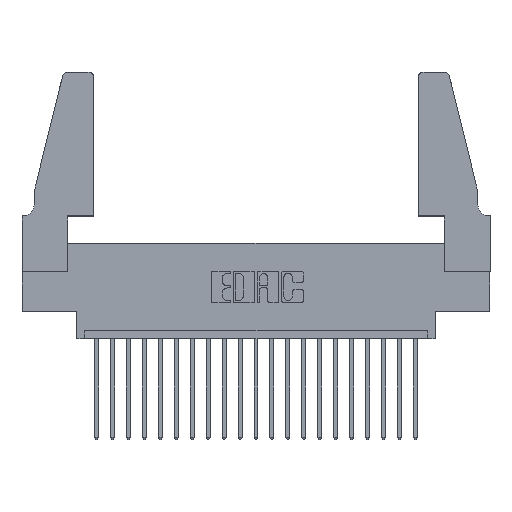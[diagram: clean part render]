
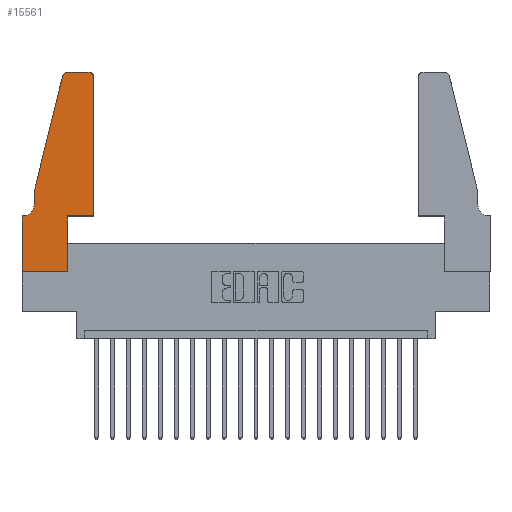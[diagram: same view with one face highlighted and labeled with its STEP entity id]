
A CAD part, top view. The second image highlights one B-rep face of the part: STEP entity #15561.
In plain terms, the highlighted planar face has unit normal (0, 0, 1).
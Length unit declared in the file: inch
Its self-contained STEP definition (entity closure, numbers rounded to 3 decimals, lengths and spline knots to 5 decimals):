
#14 = FACE_OUTER_BOUND ( 'NONE', #16671, .T. ) ;
#288 = CARTESIAN_POINT ( 'NONE',  ( 0., 0., 0.37 ) ) ;
#411 = VERTEX_POINT ( 'NONE', #14215 ) ;
#763 = EDGE_CURVE ( 'NONE', #1324, #10834, #10234, .T. ) ;
#922 = VECTOR ( 'NONE', #19363, 39.37008 ) ;
#1069 = VECTOR ( 'NONE', #16514, 39.37008 ) ;
#1324 = VERTEX_POINT ( 'NONE', #14878 ) ;
#1647 = DIRECTION ( 'NONE',  ( 0., -1., 0. ) ) ;
#1745 = DIRECTION ( 'NONE',  ( 0., 0., 1. ) ) ;
#1915 = DIRECTION ( 'NONE',  ( 1., 0., 0. ) ) ;
#1944 = ORIENTED_EDGE ( 'NONE', *, *, #763, .T. ) ;
#2121 = DIRECTION ( 'NONE',  ( 0., 0., -1. ) ) ;
#2339 = EDGE_CURVE ( 'NONE', #411, #6977, #4981, .T. ) ;
#2357 = CARTESIAN_POINT ( 'NONE',  ( 0.0755, 0.35, 0.37 ) ) ;
#2499 = ORIENTED_EDGE ( 'NONE', *, *, #9506, .T. ) ;
#2658 = ORIENTED_EDGE ( 'NONE', *, *, #4886, .T. ) ;
#2689 = CARTESIAN_POINT ( 'NONE',  ( 0.4205, 1.22, 0.37 ) ) ;
#3113 = VECTOR ( 'NONE', #1647, 39.37008 ) ;
#3152 = CIRCLE ( 'NONE', #9971, 0.03 ) ;
#3331 = DIRECTION ( 'NONE',  ( -1., 0., 0. ) ) ;
#3365 = CIRCLE ( 'NONE', #14687, 0.03 ) ;
#3493 = DIRECTION ( 'NONE',  ( 0., -1., 0. ) ) ;
#3897 = ORIENTED_EDGE ( 'NONE', *, *, #10611, .T. ) ;
#3957 = LINE ( 'NONE', #11464, #922 ) ;
#4036 = LINE ( 'NONE', #2357, #15236 ) ;
#4206 = VERTEX_POINT ( 'NONE', #18642 ) ;
#4477 = ORIENTED_EDGE ( 'NONE', *, *, #12976, .T. ) ;
#4507 = VERTEX_POINT ( 'NONE', #16225 ) ;
#4637 = EDGE_CURVE ( 'NONE', #10834, #4507, #16852, .T. ) ;
#4656 = DIRECTION ( 'NONE',  ( -1., 0., 0. ) ) ;
#4687 = ORIENTED_EDGE ( 'NONE', *, *, #18938, .T. ) ;
#4770 = CARTESIAN_POINT ( 'NONE',  ( 0., 0.35, 0.37 ) ) ;
#4886 = EDGE_CURVE ( 'NONE', #4206, #8396, #3365, .T. ) ;
#4981 = CIRCLE ( 'NONE', #7730, 0.07 ) ;
#5059 = CARTESIAN_POINT ( 'NONE',  ( 0.2865, 0., 0.37 ) ) ;
#5450 = VECTOR ( 'NONE', #19411, 39.37008 ) ;
#5942 = DIRECTION ( 'NONE',  ( 1., 0., 0. ) ) ;
#6318 = CARTESIAN_POINT ( 'NONE',  ( 0.284, 1.22, 0.37 ) ) ;
#6437 = PLANE ( 'NONE',  #16159 ) ;
#6472 = LINE ( 'NONE', #11376, #5450 ) ;
#6556 = DIRECTION ( 'NONE',  ( 0., 1., 0. ) ) ;
#6845 = CARTESIAN_POINT ( 'NONE',  ( 0.0755, 0.5, 0.37 ) ) ;
#6977 = VERTEX_POINT ( 'NONE', #12449 ) ;
#7044 = CARTESIAN_POINT ( 'NONE',  ( 0., 0.35, 0.37 ) ) ;
#7730 = AXIS2_PLACEMENT_3D ( 'NONE', #11514, #2121, #4656 ) ;
#7731 = VECTOR ( 'NONE', #6556, 39.37008 ) ;
#8396 = VERTEX_POINT ( 'NONE', #16308 ) ;
#8478 = LINE ( 'NONE', #6845, #3113 ) ;
#9409 = ORIENTED_EDGE ( 'NONE', *, *, #4637, .T. ) ;
#9506 = EDGE_CURVE ( 'NONE', #6977, #15412, #4036, .T. ) ;
#9590 = LINE ( 'NONE', #17860, #13404 ) ;
#9971 = AXIS2_PLACEMENT_3D ( 'NONE', #2689, #15674, #5942 ) ;
#10210 = DIRECTION ( 'NONE',  ( 1., 0., 0. ) ) ;
#10234 = LINE ( 'NONE', #14750, #1069 ) ;
#10611 = EDGE_CURVE ( 'NONE', #15412, #11707, #9590, .T. ) ;
#10834 = VERTEX_POINT ( 'NONE', #11887 ) ;
#11376 = CARTESIAN_POINT ( 'NONE',  ( 0.0755, 0.5, 0.37 ) ) ;
#11464 = CARTESIAN_POINT ( 'NONE',  ( 0.2865, 0.35, 0.37 ) ) ;
#11514 = CARTESIAN_POINT ( 'NONE',  ( 0.0055, 0.42, 0.37 ) ) ;
#11580 = ORIENTED_EDGE ( 'NONE', *, *, #17772, .T. ) ;
#11686 = ORIENTED_EDGE ( 'NONE', *, *, #12590, .T. ) ;
#11707 = VERTEX_POINT ( 'NONE', #20818 ) ;
#11887 = CARTESIAN_POINT ( 'NONE',  ( 0.4505, 0.35, 0.37 ) ) ;
#12279 = VERTEX_POINT ( 'NONE', #20130 ) ;
#12449 = CARTESIAN_POINT ( 'NONE',  ( 0.0055, 0.35, 0.37 ) ) ;
#12590 = EDGE_CURVE ( 'NONE', #20520, #411, #8478, .T. ) ;
#12976 = EDGE_CURVE ( 'NONE', #11707, #19196, #13339, .T. ) ;
#13339 = LINE ( 'NONE', #288, #15605 ) ;
#13404 = VECTOR ( 'NONE', #3493, 39.37008 ) ;
#14215 = CARTESIAN_POINT ( 'NONE',  ( 0.0755, 0.42, 0.37 ) ) ;
#14362 = DIRECTION ( 'NONE',  ( 0., 0., 1. ) ) ;
#14687 = AXIS2_PLACEMENT_3D ( 'NONE', #6318, #14362, #17653 ) ;
#14750 = CARTESIAN_POINT ( 'NONE',  ( 0.4505, 0.35, 0.37 ) ) ;
#14878 = CARTESIAN_POINT ( 'NONE',  ( 0.2865, 0.35, 0.37 ) ) ;
#15236 = VECTOR ( 'NONE', #17280, 39.37008 ) ;
#15412 = VERTEX_POINT ( 'NONE', #7044 ) ;
#15561 = ADVANCED_FACE ( 'NONE', ( #14 ), #6437, .T. ) ;
#15605 = VECTOR ( 'NONE', #1915, 39.37008 ) ;
#15674 = DIRECTION ( 'NONE',  ( 0., 0., 1. ) ) ;
#15897 = VECTOR ( 'NONE', #3331, 39.37008 ) ;
#16159 = AXIS2_PLACEMENT_3D ( 'NONE', #4770, #1745, #10210 ) ;
#16225 = CARTESIAN_POINT ( 'NONE',  ( 0.4505, 1.22, 0.37 ) ) ;
#16308 = CARTESIAN_POINT ( 'NONE',  ( 0.25487, 1.22718, 0.37 ) ) ;
#16514 = DIRECTION ( 'NONE',  ( 1., 0., 0. ) ) ;
#16671 = EDGE_LOOP ( 'NONE', ( #11580, #2658, #4687, #11686, #20565, #2499, #3897, #4477, #19554, #1944, #9409, #20773 ) ) ;
#16852 = LINE ( 'NONE', #17677, #7731 ) ;
#16927 = CARTESIAN_POINT ( 'NONE',  ( 0.0755, 0.5, 0.37 ) ) ;
#17280 = DIRECTION ( 'NONE',  ( -1., 0., 0. ) ) ;
#17644 = LINE ( 'NONE', #18081, #15897 ) ;
#17653 = DIRECTION ( 'NONE',  ( 1., 0., 0. ) ) ;
#17677 = CARTESIAN_POINT ( 'NONE',  ( 0.4505, 0.35, 0.37 ) ) ;
#17772 = EDGE_CURVE ( 'NONE', #12279, #4206, #17644, .T. ) ;
#17860 = CARTESIAN_POINT ( 'NONE',  ( 0., 0., 0.37 ) ) ;
#18081 = CARTESIAN_POINT ( 'NONE',  ( 0.2605, 1.25, 0.37 ) ) ;
#18258 = EDGE_CURVE ( 'NONE', #4507, #12279, #3152, .T. ) ;
#18642 = CARTESIAN_POINT ( 'NONE',  ( 0.284, 1.25, 0.37 ) ) ;
#18938 = EDGE_CURVE ( 'NONE', #8396, #20520, #6472, .T. ) ;
#19196 = VERTEX_POINT ( 'NONE', #5059 ) ;
#19232 = EDGE_CURVE ( 'NONE', #19196, #1324, #3957, .T. ) ;
#19363 = DIRECTION ( 'NONE',  ( 0., 1., 0. ) ) ;
#19411 = DIRECTION ( 'NONE',  ( -0.239, -0.971, 0. ) ) ;
#19554 = ORIENTED_EDGE ( 'NONE', *, *, #19232, .T. ) ;
#20130 = CARTESIAN_POINT ( 'NONE',  ( 0.4205, 1.25, 0.37 ) ) ;
#20520 = VERTEX_POINT ( 'NONE', #16927 ) ;
#20565 = ORIENTED_EDGE ( 'NONE', *, *, #2339, .T. ) ;
#20773 = ORIENTED_EDGE ( 'NONE', *, *, #18258, .T. ) ;
#20818 = CARTESIAN_POINT ( 'NONE',  ( 0., 0., 0.37 ) ) ;
